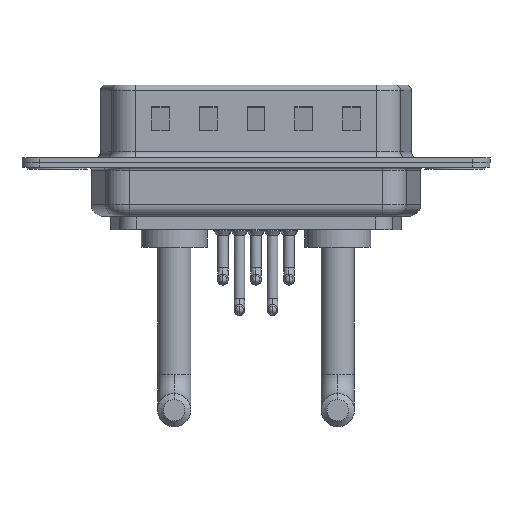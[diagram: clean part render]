
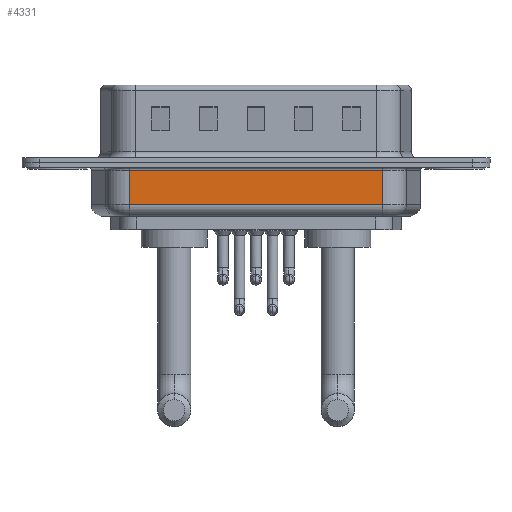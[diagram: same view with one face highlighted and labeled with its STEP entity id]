
A CAD part, front view. The second image highlights one B-rep face of the part: STEP entity #4331.
In plain terms, the highlighted planar face has unit normal (0, -1, 0).
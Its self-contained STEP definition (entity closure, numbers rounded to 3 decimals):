
#156 = CARTESIAN_POINT ( 'NONE',  ( 6.031, -5.35, -0.65 ) ) ;
#191 = CARTESIAN_POINT ( 'NONE',  ( 6.031, -5.35, -0.65 ) ) ;
#730 = VECTOR ( 'NONE', #16341, 1000. ) ;
#895 = ORIENTED_EDGE ( 'NONE', *, *, #17797, .F. ) ;
#1061 = VERTEX_POINT ( 'NONE', #156 ) ;
#1899 = LINE ( 'NONE', #191, #16663 ) ;
#3102 = EDGE_LOOP ( 'NONE', ( #895, #11946, #3828, #6757 ) ) ;
#3828 = ORIENTED_EDGE ( 'NONE', *, *, #6591, .T. ) ;
#3997 = CARTESIAN_POINT ( 'NONE',  ( 6.031, -5.35, -3.5 ) ) ;
#4331 = ADVANCED_FACE ( 'NONE', ( #8917 ), #18110, .F. ) ;
#4749 = DIRECTION ( 'NONE',  ( 0., 0., 1. ) ) ;
#5962 = LINE ( 'NONE', #14791, #730 ) ;
#6044 = EDGE_CURVE ( 'NONE', #12384, #1061, #1899, .T. ) ;
#6591 = EDGE_CURVE ( 'NONE', #7275, #12384, #5962, .T. ) ;
#6757 = ORIENTED_EDGE ( 'NONE', *, *, #6044, .T. ) ;
#7164 = LINE ( 'NONE', #9890, #17272 ) ;
#7275 = VERTEX_POINT ( 'NONE', #18530 ) ;
#7360 = CARTESIAN_POINT ( 'NONE',  ( 6.031, -5.35, -4.5 ) ) ;
#7647 = DIRECTION ( 'NONE',  ( 0., 1., 0. ) ) ;
#7712 = CARTESIAN_POINT ( 'NONE',  ( 6.031, -5.35, -4.5 ) ) ;
#8917 = FACE_OUTER_BOUND ( 'NONE', #3102, .T. ) ;
#9345 = DIRECTION ( 'NONE',  ( 0., 0., 1. ) ) ;
#9890 = CARTESIAN_POINT ( 'NONE',  ( 6.031, -5.35, -3.5 ) ) ;
#10270 = AXIS2_PLACEMENT_3D ( 'NONE', #7360, #7647, #4749 ) ;
#10722 = LINE ( 'NONE', #7712, #11633 ) ;
#10733 = DIRECTION ( 'NONE',  ( -1., 0., 0. ) ) ;
#11627 = DIRECTION ( 'NONE',  ( 1., 0., 0. ) ) ;
#11633 = VECTOR ( 'NONE', #9345, 1000. ) ;
#11946 = ORIENTED_EDGE ( 'NONE', *, *, #18970, .T. ) ;
#12384 = VERTEX_POINT ( 'NONE', #13747 ) ;
#12609 = VERTEX_POINT ( 'NONE', #3997 ) ;
#13747 = CARTESIAN_POINT ( 'NONE',  ( 27.269, -5.35, -0.65 ) ) ;
#14791 = CARTESIAN_POINT ( 'NONE',  ( 27.269, -5.35, -4.5 ) ) ;
#16341 = DIRECTION ( 'NONE',  ( 0., 0., 1. ) ) ;
#16663 = VECTOR ( 'NONE', #10733, 1000. ) ;
#17272 = VECTOR ( 'NONE', #11627, 1000. ) ;
#17797 = EDGE_CURVE ( 'NONE', #12609, #1061, #10722, .T. ) ;
#18110 = PLANE ( 'NONE',  #10270 ) ;
#18530 = CARTESIAN_POINT ( 'NONE',  ( 27.269, -5.35, -3.5 ) ) ;
#18970 = EDGE_CURVE ( 'NONE', #12609, #7275, #7164, .T. ) ;
